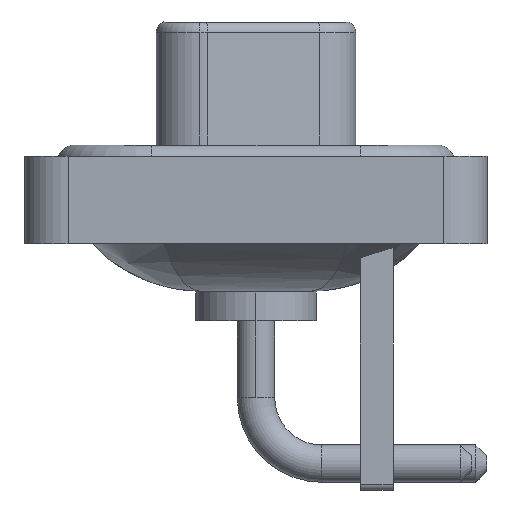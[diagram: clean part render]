
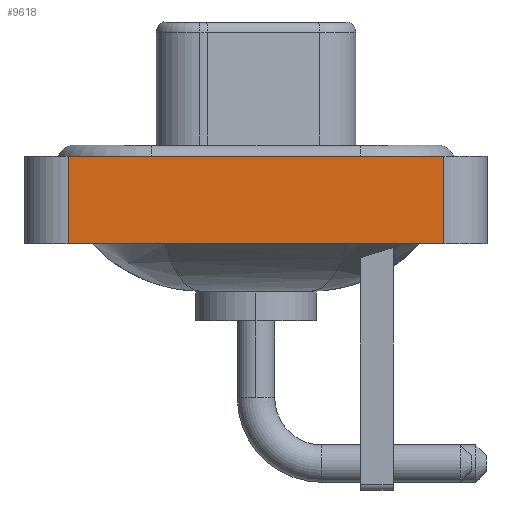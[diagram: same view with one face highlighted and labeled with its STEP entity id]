
A CAD part, left-side view. The second image highlights one B-rep face of the part: STEP entity #9618.
In plain terms, the highlighted planar face has unit normal (-1, 0, 0).
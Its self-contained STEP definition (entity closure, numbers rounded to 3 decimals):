
#188 = CARTESIAN_POINT ( 'NONE',  ( -7.3, -8.55, -3.6 ) ) ;
#861 = ORIENTED_EDGE ( 'NONE', *, *, #4259, .F. ) ;
#947 = AXIS2_PLACEMENT_3D ( 'NONE', #10312, #9919, #10214 ) ;
#1431 = CARTESIAN_POINT ( 'NONE',  ( -7.3, 8.55, -3.6 ) ) ;
#1823 = EDGE_CURVE ( 'NONE', #19178, #16106, #4070, .T. ) ;
#2560 = CARTESIAN_POINT ( 'NONE',  ( -7.3, -8.55, 0.4 ) ) ;
#4070 = LINE ( 'NONE', #14925, #11935 ) ;
#4259 = EDGE_CURVE ( 'NONE', #7865, #15946, #10147, .T. ) ;
#4538 = DIRECTION ( 'NONE',  ( 0., 0., 1. ) ) ;
#4544 = CARTESIAN_POINT ( 'NONE',  ( -7.3, -8.55, 0.4 ) ) ;
#5491 = DIRECTION ( 'NONE',  ( 0., -1., 0. ) ) ;
#5940 = ORIENTED_EDGE ( 'NONE', *, *, #11062, .F. ) ;
#6157 = LINE ( 'NONE', #13860, #9995 ) ;
#6832 = EDGE_CURVE ( 'NONE', #16106, #15946, #6157, .T. ) ;
#6986 = FACE_OUTER_BOUND ( 'NONE', #7238, .T. ) ;
#7238 = EDGE_LOOP ( 'NONE', ( #15544, #861, #5940, #10254 ) ) ;
#7472 = CARTESIAN_POINT ( 'NONE',  ( -7.3, 8.55, -3.6 ) ) ;
#7865 = VERTEX_POINT ( 'NONE', #14534 ) ;
#9618 = ADVANCED_FACE ( 'NONE', ( #6986 ), #14795, .T. ) ;
#9919 = DIRECTION ( 'NONE',  ( -1., 0., 0. ) ) ;
#9995 = VECTOR ( 'NONE', #11033, 1000. ) ;
#10147 = LINE ( 'NONE', #2560, #13574 ) ;
#10214 = DIRECTION ( 'NONE',  ( 0., 0., 1. ) ) ;
#10254 = ORIENTED_EDGE ( 'NONE', *, *, #1823, .T. ) ;
#10312 = CARTESIAN_POINT ( 'NONE',  ( -7.3, -8.55, -3.6 ) ) ;
#11033 = DIRECTION ( 'NONE',  ( 0., 0., 1. ) ) ;
#11062 = EDGE_CURVE ( 'NONE', #19178, #7865, #18334, .T. ) ;
#11935 = VECTOR ( 'NONE', #5491, 1000. ) ;
#13574 = VECTOR ( 'NONE', #15398, 1000. ) ;
#13845 = VECTOR ( 'NONE', #4538, 1000. ) ;
#13860 = CARTESIAN_POINT ( 'NONE',  ( -7.3, -8.55, -3.6 ) ) ;
#14534 = CARTESIAN_POINT ( 'NONE',  ( -7.3, 8.55, 0.4 ) ) ;
#14795 = PLANE ( 'NONE',  #947 ) ;
#14925 = CARTESIAN_POINT ( 'NONE',  ( -7.3, -8.55, -3.6 ) ) ;
#15398 = DIRECTION ( 'NONE',  ( 0., -1., 0. ) ) ;
#15544 = ORIENTED_EDGE ( 'NONE', *, *, #6832, .T. ) ;
#15946 = VERTEX_POINT ( 'NONE', #4544 ) ;
#16106 = VERTEX_POINT ( 'NONE', #188 ) ;
#18334 = LINE ( 'NONE', #7472, #13845 ) ;
#19178 = VERTEX_POINT ( 'NONE', #1431 ) ;
